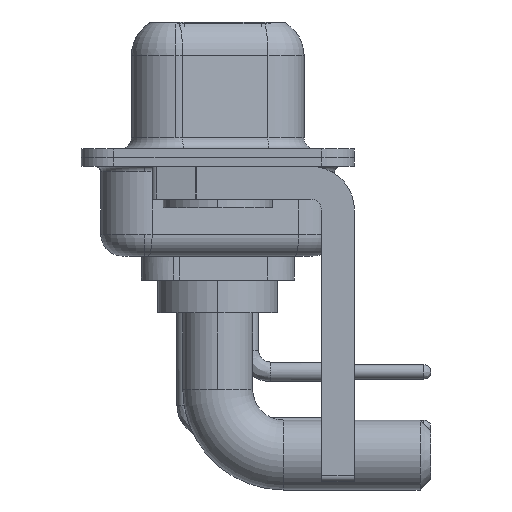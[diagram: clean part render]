
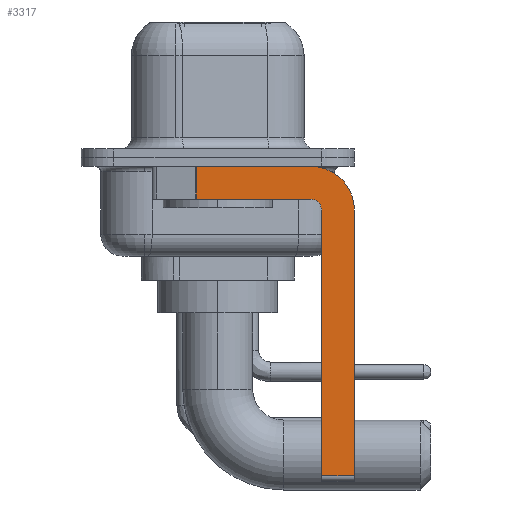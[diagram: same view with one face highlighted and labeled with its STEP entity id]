
A CAD part, left-side view. The second image highlights one B-rep face of the part: STEP entity #3317.
In plain terms, the highlighted planar face has unit normal (-1, 0, 0).
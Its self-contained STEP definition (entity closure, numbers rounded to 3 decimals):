
#143 = CARTESIAN_POINT ( 'NONE',  ( -2.9, 0.978, -1.9 ) ) ;
#380 = VERTEX_POINT ( 'NONE', #17040 ) ;
#879 = EDGE_CURVE ( 'NONE', #11095, #7777, #6220, .T. ) ;
#1109 = DIRECTION ( 'NONE',  ( 1., 0., 0. ) ) ;
#1137 = CARTESIAN_POINT ( 'NONE',  ( -2.9, -4.75, -2.4 ) ) ;
#1177 = DIRECTION ( 'NONE',  ( 1., 0., 0. ) ) ;
#1456 = DIRECTION ( 'NONE',  ( 0., 1., 0. ) ) ;
#1496 = ORIENTED_EDGE ( 'NONE', *, *, #18139, .F. ) ;
#1646 = LINE ( 'NONE', #3351, #19594 ) ;
#1665 = LINE ( 'NONE', #10701, #4527 ) ;
#2239 = ORIENTED_EDGE ( 'NONE', *, *, #16935, .T. ) ;
#2349 = EDGE_CURVE ( 'NONE', #3257, #4536, #13184, .T. ) ;
#2492 = CARTESIAN_POINT ( 'NONE',  ( -2.9, -4.25, -14.55 ) ) ;
#2560 = DIRECTION ( 'NONE',  ( 0., 0., 1. ) ) ;
#3115 = DIRECTION ( 'NONE',  ( 0., 0., -1. ) ) ;
#3257 = VERTEX_POINT ( 'NONE', #4194 ) ;
#3317 = ADVANCED_FACE ( 'NONE', ( #12111 ), #13420, .F. ) ;
#3351 = CARTESIAN_POINT ( 'NONE',  ( -2.9, 3., -0.4 ) ) ;
#3478 = ORIENTED_EDGE ( 'NONE', *, *, #15139, .F. ) ;
#3981 = DIRECTION ( 'NONE',  ( 0., 0., -1. ) ) ;
#4142 = CARTESIAN_POINT ( 'NONE',  ( -2.9, -4.75, -14.8 ) ) ;
#4194 = CARTESIAN_POINT ( 'NONE',  ( -2.9, -4.25, -0.4 ) ) ;
#4221 = VECTOR ( 'NONE', #19328, 1000. ) ;
#4395 = DIRECTION ( 'NONE',  ( 0., 0., -1. ) ) ;
#4527 = VECTOR ( 'NONE', #16702, 1000. ) ;
#4536 = VERTEX_POINT ( 'NONE', #17372 ) ;
#4848 = AXIS2_PLACEMENT_3D ( 'NONE', #11705, #1177, #3981 ) ;
#5056 = ORIENTED_EDGE ( 'NONE', *, *, #19376, .F. ) ;
#5389 = ORIENTED_EDGE ( 'NONE', *, *, #10808, .F. ) ;
#5909 = CARTESIAN_POINT ( 'NONE',  ( -2.9, -4.25, -2.4 ) ) ;
#6220 = LINE ( 'NONE', #16852, #7253 ) ;
#7070 = CARTESIAN_POINT ( 'NONE',  ( -2.9, -4.25, -2.4 ) ) ;
#7087 = VERTEX_POINT ( 'NONE', #19632 ) ;
#7253 = VECTOR ( 'NONE', #3115, 1000. ) ;
#7777 = VERTEX_POINT ( 'NONE', #143 ) ;
#7995 = EDGE_LOOP ( 'NONE', ( #1496, #8505, #5056, #3478, #5389, #2239, #12262, #8253 ) ) ;
#8253 = ORIENTED_EDGE ( 'NONE', *, *, #2349, .F. ) ;
#8505 = ORIENTED_EDGE ( 'NONE', *, *, #879, .T. ) ;
#9875 = DIRECTION ( 'NONE',  ( -1., 0., 0. ) ) ;
#10221 = CARTESIAN_POINT ( 'NONE',  ( -2.9, -4.25, -1.9 ) ) ;
#10406 = EDGE_CURVE ( 'NONE', #4536, #380, #1665, .T. ) ;
#10701 = CARTESIAN_POINT ( 'NONE',  ( -2.9, -6.25, -2.4 ) ) ;
#10808 = EDGE_CURVE ( 'NONE', #16905, #12669, #17893, .T. ) ;
#11095 = VERTEX_POINT ( 'NONE', #18581 ) ;
#11705 = CARTESIAN_POINT ( 'NONE',  ( -2.9, -4.25, -2.4 ) ) ;
#11939 = AXIS2_PLACEMENT_3D ( 'NONE', #5909, #1109, #4395 ) ;
#12111 = FACE_OUTER_BOUND ( 'NONE', #7995, .T. ) ;
#12260 = VECTOR ( 'NONE', #1456, 1000. ) ;
#12262 = ORIENTED_EDGE ( 'NONE', *, *, #10406, .F. ) ;
#12669 = VERTEX_POINT ( 'NONE', #1137 ) ;
#13046 = DIRECTION ( 'NONE',  ( 0., -1., 0. ) ) ;
#13184 = CIRCLE ( 'NONE', #4848, 2. ) ;
#13420 = PLANE ( 'NONE',  #11939 ) ;
#13734 = CARTESIAN_POINT ( 'NONE',  ( -2.9, -4.75, -14.55 ) ) ;
#15139 = EDGE_CURVE ( 'NONE', #12669, #7087, #16514, .T. ) ;
#16314 = LINE ( 'NONE', #10221, #12260 ) ;
#16378 = DIRECTION ( 'NONE',  ( 0., 0., 1. ) ) ;
#16514 = CIRCLE ( 'NONE', #19070, 0.5 ) ;
#16702 = DIRECTION ( 'NONE',  ( 0., 0., -1. ) ) ;
#16852 = CARTESIAN_POINT ( 'NONE',  ( -2.9, 0.978, -1.9 ) ) ;
#16905 = VERTEX_POINT ( 'NONE', #13734 ) ;
#16935 = EDGE_CURVE ( 'NONE', #16905, #380, #17723, .T. ) ;
#17040 = CARTESIAN_POINT ( 'NONE',  ( -2.9, -6.25, -14.55 ) ) ;
#17372 = CARTESIAN_POINT ( 'NONE',  ( -2.9, -6.25, -2.4 ) ) ;
#17723 = LINE ( 'NONE', #2492, #4221 ) ;
#17893 = LINE ( 'NONE', #4142, #18016 ) ;
#18016 = VECTOR ( 'NONE', #16378, 1000. ) ;
#18139 = EDGE_CURVE ( 'NONE', #11095, #3257, #1646, .T. ) ;
#18581 = CARTESIAN_POINT ( 'NONE',  ( -2.9, 0.978, -0.4 ) ) ;
#19070 = AXIS2_PLACEMENT_3D ( 'NONE', #7070, #9875, #2560 ) ;
#19328 = DIRECTION ( 'NONE',  ( 0., -1., 0. ) ) ;
#19376 = EDGE_CURVE ( 'NONE', #7087, #7777, #16314, .T. ) ;
#19594 = VECTOR ( 'NONE', #13046, 1000. ) ;
#19632 = CARTESIAN_POINT ( 'NONE',  ( -2.9, -4.25, -1.9 ) ) ;
